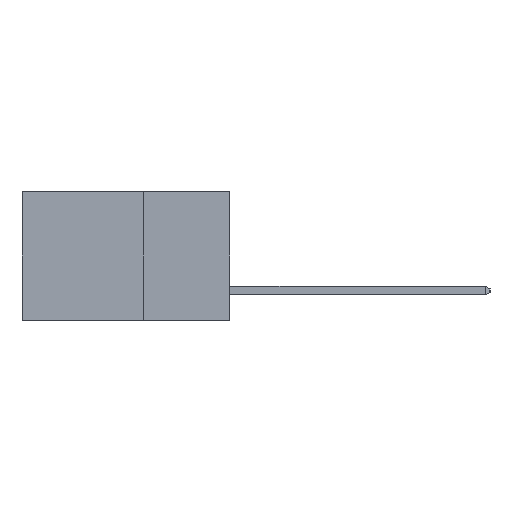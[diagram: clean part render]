
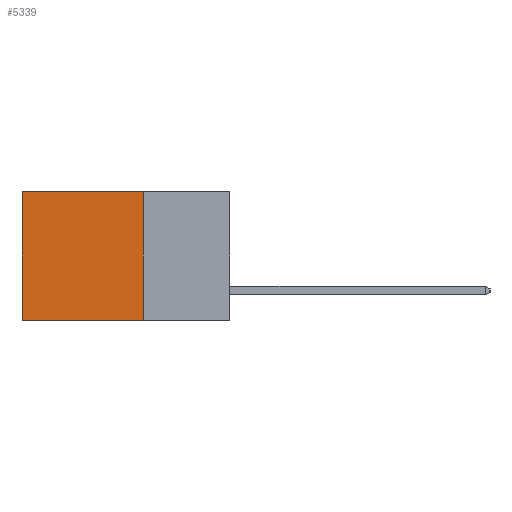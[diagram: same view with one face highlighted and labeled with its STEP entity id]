
A CAD part, left-side view. The second image highlights one B-rep face of the part: STEP entity #5339.
In plain terms, the highlighted planar face has unit normal (-1, 0, 0).
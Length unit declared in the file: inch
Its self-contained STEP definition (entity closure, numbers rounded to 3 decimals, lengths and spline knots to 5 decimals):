
#34 = ORIENTED_EDGE ( 'NONE', *, *, #4541, .T. ) ;
#1591 = CARTESIAN_POINT ( 'NONE',  ( 0.298, 0.25, 0. ) ) ;
#1926 = VECTOR ( 'NONE', #14909, 39.37008 ) ;
#2338 = CARTESIAN_POINT ( 'NONE',  ( 0.298, 0.25, 0. ) ) ;
#2965 = CARTESIAN_POINT ( 'NONE',  ( 0.298, 0.25, -0.37 ) ) ;
#3529 = DIRECTION ( 'NONE',  ( 0., 0., -1. ) ) ;
#3942 = VECTOR ( 'NONE', #5061, 39.37008 ) ;
#4037 = CARTESIAN_POINT ( 'NONE',  ( 0.298, 0.6, -0.37 ) ) ;
#4283 = FACE_OUTER_BOUND ( 'NONE', #6023, .T. ) ;
#4541 = EDGE_CURVE ( 'NONE', #7001, #5481, #5390, .T. ) ;
#5061 = DIRECTION ( 'NONE',  ( 0., 0., -1. ) ) ;
#5339 = ADVANCED_FACE ( 'NONE', ( #4283 ), #10312, .F. ) ;
#5390 = LINE ( 'NONE', #1591, #1926 ) ;
#5481 = VERTEX_POINT ( 'NONE', #11830 ) ;
#5924 = CARTESIAN_POINT ( 'NONE',  ( 0.298, 0.25, 0. ) ) ;
#5998 = EDGE_CURVE ( 'NONE', #10437, #9012, #12230, .T. ) ;
#6023 = EDGE_LOOP ( 'NONE', ( #9097, #9231, #9111, #34 ) ) ;
#6996 = LINE ( 'NONE', #2338, #12815 ) ;
#7001 = VERTEX_POINT ( 'NONE', #5924 ) ;
#7345 = LINE ( 'NONE', #8526, #3942 ) ;
#7427 = EDGE_CURVE ( 'NONE', #7001, #10437, #6996, .T. ) ;
#8526 = CARTESIAN_POINT ( 'NONE',  ( 0.298, 0.6, 0. ) ) ;
#9012 = VERTEX_POINT ( 'NONE', #4037 ) ;
#9097 = ORIENTED_EDGE ( 'NONE', *, *, #10238, .T. ) ;
#9111 = ORIENTED_EDGE ( 'NONE', *, *, #7427, .F. ) ;
#9139 = VECTOR ( 'NONE', #14475, 39.37008 ) ;
#9231 = ORIENTED_EDGE ( 'NONE', *, *, #5998, .F. ) ;
#10013 = CARTESIAN_POINT ( 'NONE',  ( 0.298, 0.25, -0.37 ) ) ;
#10238 = EDGE_CURVE ( 'NONE', #5481, #9012, #7345, .T. ) ;
#10312 = PLANE ( 'NONE',  #10458 ) ;
#10437 = VERTEX_POINT ( 'NONE', #10013 ) ;
#10458 = AXIS2_PLACEMENT_3D ( 'NONE', #13989, #13742, #13726 ) ;
#11830 = CARTESIAN_POINT ( 'NONE',  ( 0.298, 0.6, 0. ) ) ;
#12230 = LINE ( 'NONE', #2965, #9139 ) ;
#12815 = VECTOR ( 'NONE', #3529, 39.37008 ) ;
#13726 = DIRECTION ( 'NONE',  ( 0., 0., -1. ) ) ;
#13742 = DIRECTION ( 'NONE',  ( 1., 0., 0. ) ) ;
#13989 = CARTESIAN_POINT ( 'NONE',  ( 0.298, 0.25, 0. ) ) ;
#14475 = DIRECTION ( 'NONE',  ( 0., 1., 0. ) ) ;
#14909 = DIRECTION ( 'NONE',  ( 0., 1., 0. ) ) ;
